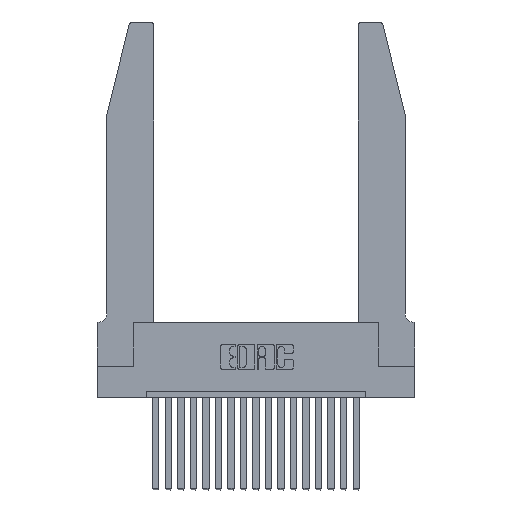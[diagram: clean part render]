
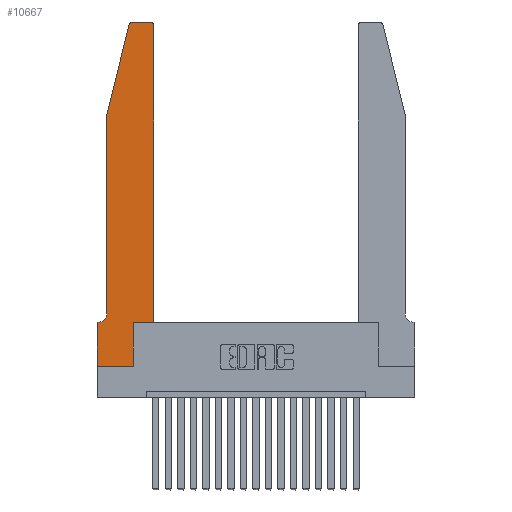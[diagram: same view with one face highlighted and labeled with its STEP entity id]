
A CAD part, top view. The second image highlights one B-rep face of the part: STEP entity #10667.
In plain terms, the highlighted planar face has unit normal (0, 0, 1).
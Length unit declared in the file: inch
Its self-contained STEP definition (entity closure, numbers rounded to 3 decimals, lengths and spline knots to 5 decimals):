
#335 = CARTESIAN_POINT ( 'NONE',  ( 0.0055, 0.35, 0.37 ) ) ;
#505 = CARTESIAN_POINT ( 'NONE',  ( 0.2865, 0.35, 0.37 ) ) ;
#610 = VERTEX_POINT ( 'NONE', #17089 ) ;
#744 = CARTESIAN_POINT ( 'NONE',  ( 0., 0.35, 0.37 ) ) ;
#992 = VERTEX_POINT ( 'NONE', #335 ) ;
#1199 = CARTESIAN_POINT ( 'NONE',  ( 0.25487, 2.72718, 0.37 ) ) ;
#1290 = EDGE_CURVE ( 'NONE', #6642, #13444, #17336, .T. ) ;
#1361 = VERTEX_POINT ( 'NONE', #1438 ) ;
#1438 = CARTESIAN_POINT ( 'NONE',  ( 0.2865, 0.35, 0.37 ) ) ;
#1628 = ORIENTED_EDGE ( 'NONE', *, *, #1290, .T. ) ;
#1659 = EDGE_CURVE ( 'NONE', #18046, #992, #18314, .T. ) ;
#2223 = VERTEX_POINT ( 'NONE', #8911 ) ;
#2259 = CARTESIAN_POINT ( 'NONE',  ( 0., 0., 0.37 ) ) ;
#2332 = DIRECTION ( 'NONE',  ( 1., 0., 0. ) ) ;
#2379 = EDGE_LOOP ( 'NONE', ( #17582, #20156, #13137, #5172, #12266, #17651, #5371, #14670, #6945, #7784, #9505, #1628 ) ) ;
#2407 = LINE ( 'NONE', #4519, #14499 ) ;
#2562 = LINE ( 'NONE', #19427, #5853 ) ;
#2761 = EDGE_CURVE ( 'NONE', #13444, #610, #8473, .T. ) ;
#2767 = DIRECTION ( 'NONE',  ( 0., -1., 0. ) ) ;
#3169 = AXIS2_PLACEMENT_3D ( 'NONE', #14896, #13095, #3457 ) ;
#3447 = DIRECTION ( 'NONE',  ( 1., 0., 0. ) ) ;
#3457 = DIRECTION ( 'NONE',  ( 1., 0., 0. ) ) ;
#3695 = VERTEX_POINT ( 'NONE', #2259 ) ;
#4146 = VECTOR ( 'NONE', #19772, 39.37008 ) ;
#4147 = LINE ( 'NONE', #10884, #4388 ) ;
#4227 = LINE ( 'NONE', #15238, #11777 ) ;
#4388 = VECTOR ( 'NONE', #12577, 39.37008 ) ;
#4519 = CARTESIAN_POINT ( 'NONE',  ( 0.4505, 0.35, 0.37 ) ) ;
#4655 = EDGE_CURVE ( 'NONE', #3695, #9374, #2562, .T. ) ;
#4988 = FACE_OUTER_BOUND ( 'NONE', #2379, .T. ) ;
#5172 = ORIENTED_EDGE ( 'NONE', *, *, #8045, .T. ) ;
#5199 = CARTESIAN_POINT ( 'NONE',  ( 0.4505, 0.35, 0.37 ) ) ;
#5371 = ORIENTED_EDGE ( 'NONE', *, *, #20267, .T. ) ;
#5572 = DIRECTION ( 'NONE',  ( -1., 0., 0. ) ) ;
#5824 = CARTESIAN_POINT ( 'NONE',  ( 0.4505, 2.72, 0.37 ) ) ;
#5853 = VECTOR ( 'NONE', #3447, 39.37008 ) ;
#5920 = VERTEX_POINT ( 'NONE', #7581 ) ;
#6194 = CIRCLE ( 'NONE', #3169, 0.03 ) ;
#6283 = LINE ( 'NONE', #19361, #7288 ) ;
#6642 = VERTEX_POINT ( 'NONE', #5824 ) ;
#6945 = ORIENTED_EDGE ( 'NONE', *, *, #13252, .T. ) ;
#7116 = DIRECTION ( 'NONE',  ( 0., 0., -1. ) ) ;
#7165 = CARTESIAN_POINT ( 'NONE',  ( 0.4205, 2.75, 0.37 ) ) ;
#7280 = AXIS2_PLACEMENT_3D ( 'NONE', #19991, #7116, #5572 ) ;
#7288 = VECTOR ( 'NONE', #2767, 39.37008 ) ;
#7581 = CARTESIAN_POINT ( 'NONE',  ( 0.4505, 0.35, 0.37 ) ) ;
#7784 = ORIENTED_EDGE ( 'NONE', *, *, #11746, .T. ) ;
#8045 = EDGE_CURVE ( 'NONE', #19515, #18046, #4227, .T. ) ;
#8085 = CARTESIAN_POINT ( 'NONE',  ( 0.0755, 0.42, 0.37 ) ) ;
#8473 = LINE ( 'NONE', #18751, #11469 ) ;
#8894 = PLANE ( 'NONE',  #14188 ) ;
#8911 = CARTESIAN_POINT ( 'NONE',  ( 0., 0.35, 0.37 ) ) ;
#9297 = LINE ( 'NONE', #5199, #13070 ) ;
#9374 = VERTEX_POINT ( 'NONE', #20431 ) ;
#9505 = ORIENTED_EDGE ( 'NONE', *, *, #9921, .T. ) ;
#9546 = CARTESIAN_POINT ( 'NONE',  ( 0.0755, 0.35, 0.37 ) ) ;
#9921 = EDGE_CURVE ( 'NONE', #5920, #6642, #9297, .T. ) ;
#10060 = DIRECTION ( 'NONE',  ( 0., 1., 0. ) ) ;
#10396 = CARTESIAN_POINT ( 'NONE',  ( 0.0755, 2., 0.37 ) ) ;
#10667 = ADVANCED_FACE ( 'NONE', ( #4988 ), #8894, .T. ) ;
#10884 = CARTESIAN_POINT ( 'NONE',  ( 0.0755, 2., 0.37 ) ) ;
#10927 = DIRECTION ( 'NONE',  ( 0., 0., 1. ) ) ;
#10932 = LINE ( 'NONE', #505, #4146 ) ;
#11469 = VECTOR ( 'NONE', #14089, 39.37008 ) ;
#11746 = EDGE_CURVE ( 'NONE', #1361, #5920, #2407, .T. ) ;
#11777 = VECTOR ( 'NONE', #20194, 39.37008 ) ;
#11893 = EDGE_CURVE ( 'NONE', #610, #17766, #6194, .T. ) ;
#11998 = DIRECTION ( 'NONE',  ( 0., 0., 1. ) ) ;
#12266 = ORIENTED_EDGE ( 'NONE', *, *, #1659, .T. ) ;
#12577 = DIRECTION ( 'NONE',  ( -0.239, -0.971, 0. ) ) ;
#13070 = VECTOR ( 'NONE', #10060, 39.37008 ) ;
#13095 = DIRECTION ( 'NONE',  ( 0., 0., 1. ) ) ;
#13137 = ORIENTED_EDGE ( 'NONE', *, *, #16519, .T. ) ;
#13252 = EDGE_CURVE ( 'NONE', #9374, #1361, #10932, .T. ) ;
#13348 = AXIS2_PLACEMENT_3D ( 'NONE', #14143, #10927, #14078 ) ;
#13444 = VERTEX_POINT ( 'NONE', #7165 ) ;
#14010 = EDGE_CURVE ( 'NONE', #992, #2223, #18638, .T. ) ;
#14078 = DIRECTION ( 'NONE',  ( 1., 0., 0. ) ) ;
#14089 = DIRECTION ( 'NONE',  ( -1., 0., 0. ) ) ;
#14143 = CARTESIAN_POINT ( 'NONE',  ( 0.4205, 2.72, 0.37 ) ) ;
#14188 = AXIS2_PLACEMENT_3D ( 'NONE', #744, #11998, #2332 ) ;
#14499 = VECTOR ( 'NONE', #17488, 39.37008 ) ;
#14670 = ORIENTED_EDGE ( 'NONE', *, *, #4655, .T. ) ;
#14896 = CARTESIAN_POINT ( 'NONE',  ( 0.284, 2.72, 0.37 ) ) ;
#15238 = CARTESIAN_POINT ( 'NONE',  ( 0.0755, 2., 0.37 ) ) ;
#16519 = EDGE_CURVE ( 'NONE', #17766, #19515, #4147, .T. ) ;
#17089 = CARTESIAN_POINT ( 'NONE',  ( 0.284, 2.75, 0.37 ) ) ;
#17336 = CIRCLE ( 'NONE', #13348, 0.03 ) ;
#17436 = DIRECTION ( 'NONE',  ( -1., 0., 0. ) ) ;
#17488 = DIRECTION ( 'NONE',  ( 1., 0., 0. ) ) ;
#17582 = ORIENTED_EDGE ( 'NONE', *, *, #2761, .T. ) ;
#17651 = ORIENTED_EDGE ( 'NONE', *, *, #14010, .T. ) ;
#17766 = VERTEX_POINT ( 'NONE', #1199 ) ;
#18046 = VERTEX_POINT ( 'NONE', #8085 ) ;
#18314 = CIRCLE ( 'NONE', #7280, 0.07 ) ;
#18638 = LINE ( 'NONE', #9546, #19407 ) ;
#18751 = CARTESIAN_POINT ( 'NONE',  ( 0.2605, 2.75, 0.37 ) ) ;
#19361 = CARTESIAN_POINT ( 'NONE',  ( 0., 0., 0.37 ) ) ;
#19407 = VECTOR ( 'NONE', #17436, 39.37008 ) ;
#19427 = CARTESIAN_POINT ( 'NONE',  ( 0., 0., 0.37 ) ) ;
#19515 = VERTEX_POINT ( 'NONE', #10396 ) ;
#19772 = DIRECTION ( 'NONE',  ( 0., 1., 0. ) ) ;
#19991 = CARTESIAN_POINT ( 'NONE',  ( 0.0055, 0.42, 0.37 ) ) ;
#20156 = ORIENTED_EDGE ( 'NONE', *, *, #11893, .T. ) ;
#20194 = DIRECTION ( 'NONE',  ( 0., -1., 0. ) ) ;
#20267 = EDGE_CURVE ( 'NONE', #2223, #3695, #6283, .T. ) ;
#20431 = CARTESIAN_POINT ( 'NONE',  ( 0.2865, 0., 0.37 ) ) ;
